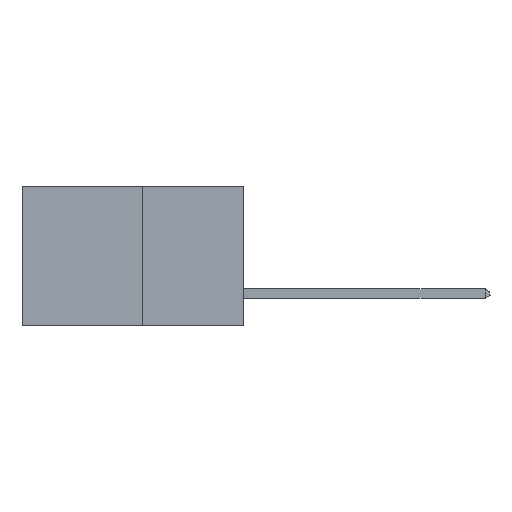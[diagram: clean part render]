
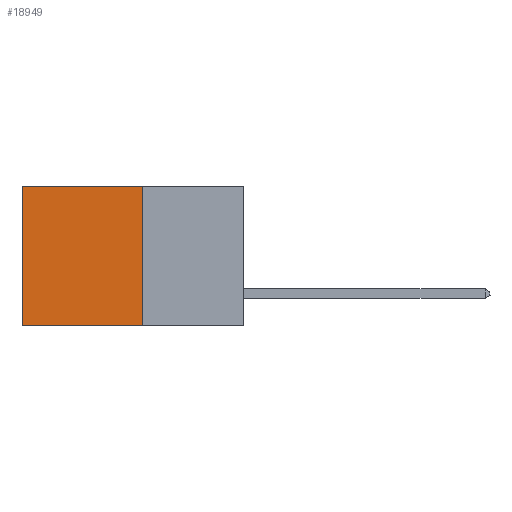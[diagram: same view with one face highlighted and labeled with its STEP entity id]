
A CAD part, left-side view. The second image highlights one B-rep face of the part: STEP entity #18949.
In plain terms, the highlighted planar face has unit normal (-1, 0, 0).
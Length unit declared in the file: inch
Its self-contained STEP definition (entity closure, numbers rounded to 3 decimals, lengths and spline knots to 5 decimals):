
#582 = VERTEX_POINT ( 'NONE', #4691 ) ;
#1082 = VERTEX_POINT ( 'NONE', #2781 ) ;
#1523 = ORIENTED_EDGE ( 'NONE', *, *, #9279, .F. ) ;
#1555 = EDGE_CURVE ( 'NONE', #1082, #582, #4933, .T. ) ;
#1842 = VECTOR ( 'NONE', #12650, 39.37008 ) ;
#2781 = CARTESIAN_POINT ( 'NONE',  ( 0.277, 0.59, 0. ) ) ;
#3375 = VERTEX_POINT ( 'NONE', #16664 ) ;
#3823 = CARTESIAN_POINT ( 'NONE',  ( 0.277, 0.27, 0. ) ) ;
#3828 = EDGE_CURVE ( 'NONE', #3375, #1082, #13620, .T. ) ;
#4691 = CARTESIAN_POINT ( 'NONE',  ( 0.277, 0.59, -0.37 ) ) ;
#4798 = CARTESIAN_POINT ( 'NONE',  ( 0.277, 0.27, -0.37 ) ) ;
#4933 = LINE ( 'NONE', #17641, #11393 ) ;
#6298 = DIRECTION ( 'NONE',  ( 0., 0., -1. ) ) ;
#6774 = ORIENTED_EDGE ( 'NONE', *, *, #17126, .F. ) ;
#7272 = AXIS2_PLACEMENT_3D ( 'NONE', #4798, #15055, #6298 ) ;
#9279 = EDGE_CURVE ( 'NONE', #15756, #582, #15174, .T. ) ;
#10667 = PLANE ( 'NONE',  #7272 ) ;
#10844 = VECTOR ( 'NONE', #13328, 39.37008 ) ;
#11278 = ORIENTED_EDGE ( 'NONE', *, *, #1555, .T. ) ;
#11393 = VECTOR ( 'NONE', #17518, 39.37008 ) ;
#12173 = DIRECTION ( 'NONE',  ( 0., 0., -1. ) ) ;
#12650 = DIRECTION ( 'NONE',  ( 0., 1., 0. ) ) ;
#13328 = DIRECTION ( 'NONE',  ( 0., 1., 0. ) ) ;
#13368 = CARTESIAN_POINT ( 'NONE',  ( 0.277, 0.27, -0.37 ) ) ;
#13620 = LINE ( 'NONE', #3823, #1842 ) ;
#13904 = EDGE_LOOP ( 'NONE', ( #11278, #1523, #6774, #18135 ) ) ;
#14523 = FACE_OUTER_BOUND ( 'NONE', #13904, .T. ) ;
#14749 = CARTESIAN_POINT ( 'NONE',  ( 0.277, 0.27, -0.37 ) ) ;
#15055 = DIRECTION ( 'NONE',  ( 1., 0., 0. ) ) ;
#15174 = LINE ( 'NONE', #14749, #10844 ) ;
#15756 = VERTEX_POINT ( 'NONE', #13368 ) ;
#16664 = CARTESIAN_POINT ( 'NONE',  ( 0.277, 0.27, 0. ) ) ;
#17126 = EDGE_CURVE ( 'NONE', #3375, #15756, #17827, .T. ) ;
#17373 = VECTOR ( 'NONE', #12173, 39.37008 ) ;
#17518 = DIRECTION ( 'NONE',  ( 0., 0., -1. ) ) ;
#17641 = CARTESIAN_POINT ( 'NONE',  ( 0.277, 0.59, -0.37 ) ) ;
#17827 = LINE ( 'NONE', #17956, #17373 ) ;
#17956 = CARTESIAN_POINT ( 'NONE',  ( 0.277, 0.27, -0.37 ) ) ;
#18135 = ORIENTED_EDGE ( 'NONE', *, *, #3828, .T. ) ;
#18949 = ADVANCED_FACE ( 'NONE', ( #14523 ), #10667, .F. ) ;
